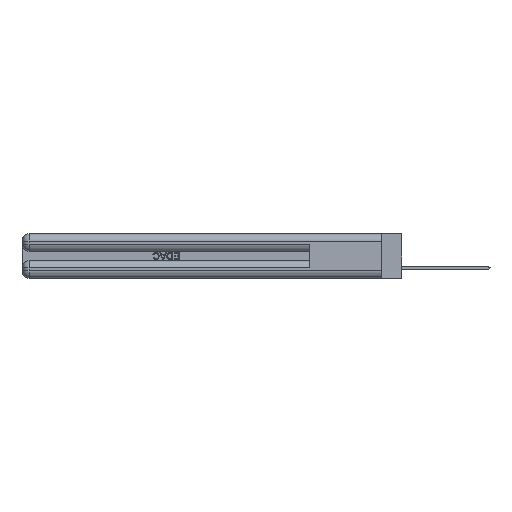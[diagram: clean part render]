
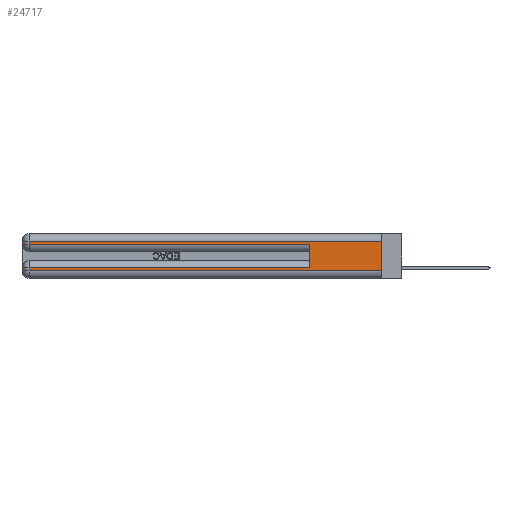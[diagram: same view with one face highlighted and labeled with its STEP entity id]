
A CAD part, left-side view. The second image highlights one B-rep face of the part: STEP entity #24717.
In plain terms, the highlighted planar face has unit normal (-1, 0, 0).
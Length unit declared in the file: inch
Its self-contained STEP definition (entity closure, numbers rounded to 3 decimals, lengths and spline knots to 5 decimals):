
#1017 = EDGE_CURVE ( 'NONE', #30338, #10760, #43060, .T. ) ;
#1776 = CARTESIAN_POINT ( 'NONE',  ( 0., 0., 0.31 ) ) ;
#2384 = CARTESIAN_POINT ( 'NONE',  ( 0., 0.6, 0.085 ) ) ;
#2623 = PLANE ( 'NONE',  #31251 ) ;
#4353 = VERTEX_POINT ( 'NONE', #27204 ) ;
#7682 = VECTOR ( 'NONE', #43996, 39.37008 ) ;
#8694 = VECTOR ( 'NONE', #31365, 39.37008 ) ;
#8896 = EDGE_LOOP ( 'NONE', ( #10251, #34363, #15253, #35273, #28475, #35552, #41959, #15795 ) ) ;
#10251 = ORIENTED_EDGE ( 'NONE', *, *, #39786, .F. ) ;
#10760 = VERTEX_POINT ( 'NONE', #42130 ) ;
#11633 = VERTEX_POINT ( 'NONE', #11650 ) ;
#11650 = CARTESIAN_POINT ( 'NONE',  ( 0., 0., 0.31 ) ) ;
#13659 = DIRECTION ( 'NONE',  ( 0., 0., -1. ) ) ;
#13691 = CARTESIAN_POINT ( 'NONE',  ( 0., 0., 0.085 ) ) ;
#13802 = VECTOR ( 'NONE', #17091, 39.37008 ) ;
#14340 = CARTESIAN_POINT ( 'NONE',  ( 0., 0., 0.06 ) ) ;
#14368 = CARTESIAN_POINT ( 'NONE',  ( 0., 0.6, 0.145 ) ) ;
#15253 = ORIENTED_EDGE ( 'NONE', *, *, #37008, .T. ) ;
#15402 = VECTOR ( 'NONE', #17909, 39.37008 ) ;
#15795 = ORIENTED_EDGE ( 'NONE', *, *, #37630, .T. ) ;
#16189 = LINE ( 'NONE', #1776, #31571 ) ;
#16237 = FACE_OUTER_BOUND ( 'NONE', #8896, .T. ) ;
#16579 = VECTOR ( 'NONE', #17939, 39.37008 ) ;
#16727 = CARTESIAN_POINT ( 'NONE',  ( 0., 0., 0.37 ) ) ;
#17091 = DIRECTION ( 'NONE',  ( 0., 1., 0. ) ) ;
#17909 = DIRECTION ( 'NONE',  ( 0., -1., 0. ) ) ;
#17939 = DIRECTION ( 'NONE',  ( 0., 0., 1. ) ) ;
#18750 = CARTESIAN_POINT ( 'NONE',  ( 0., 2.94, 0.37 ) ) ;
#20159 = VECTOR ( 'NONE', #25986, 39.37008 ) ;
#20836 = LINE ( 'NONE', #38506, #8694 ) ;
#21003 = EDGE_CURVE ( 'NONE', #36018, #32308, #36309, .T. ) ;
#21335 = CARTESIAN_POINT ( 'NONE',  ( 0., 2.94, 0.085 ) ) ;
#22274 = DIRECTION ( 'NONE',  ( 0., 0., -1. ) ) ;
#22298 = CARTESIAN_POINT ( 'NONE',  ( 0., 0., 0.285 ) ) ;
#22446 = CARTESIAN_POINT ( 'NONE',  ( 0., 2.94, 0.285 ) ) ;
#24717 = ADVANCED_FACE ( 'NONE', ( #16237 ), #2623, .F. ) ;
#24850 = VECTOR ( 'NONE', #22274, 39.37008 ) ;
#25943 = VERTEX_POINT ( 'NONE', #22446 ) ;
#25986 = DIRECTION ( 'NONE',  ( 0., 0., -1. ) ) ;
#27204 = CARTESIAN_POINT ( 'NONE',  ( 0., 2.94, 0.31 ) ) ;
#27719 = VERTEX_POINT ( 'NONE', #33353 ) ;
#27754 = EDGE_CURVE ( 'NONE', #25943, #32308, #35657, .T. ) ;
#28475 = ORIENTED_EDGE ( 'NONE', *, *, #21003, .F. ) ;
#28573 = CARTESIAN_POINT ( 'NONE',  ( 0., 2.94, 0.37 ) ) ;
#30338 = VERTEX_POINT ( 'NONE', #21335 ) ;
#31251 = AXIS2_PLACEMENT_3D ( 'NONE', #16727, #44143, #13659 ) ;
#31365 = DIRECTION ( 'NONE',  ( 0., 0., -1. ) ) ;
#31571 = VECTOR ( 'NONE', #36596, 39.37008 ) ;
#31593 = EDGE_CURVE ( 'NONE', #36018, #30338, #39519, .T. ) ;
#32308 = VERTEX_POINT ( 'NONE', #41978 ) ;
#33353 = CARTESIAN_POINT ( 'NONE',  ( 0., 0., 0.06 ) ) ;
#34186 = LINE ( 'NONE', #18750, #24850 ) ;
#34363 = ORIENTED_EDGE ( 'NONE', *, *, #43766, .T. ) ;
#35273 = ORIENTED_EDGE ( 'NONE', *, *, #27754, .T. ) ;
#35552 = ORIENTED_EDGE ( 'NONE', *, *, #31593, .T. ) ;
#35657 = LINE ( 'NONE', #22298, #7682 ) ;
#36018 = VERTEX_POINT ( 'NONE', #2384 ) ;
#36309 = LINE ( 'NONE', #14368, #16579 ) ;
#36596 = DIRECTION ( 'NONE',  ( 0., 1., 0. ) ) ;
#37008 = EDGE_CURVE ( 'NONE', #4353, #25943, #34186, .T. ) ;
#37630 = EDGE_CURVE ( 'NONE', #10760, #27719, #37937, .T. ) ;
#37937 = LINE ( 'NONE', #14340, #15402 ) ;
#38506 = CARTESIAN_POINT ( 'NONE',  ( 0., 0., 0.37 ) ) ;
#39519 = LINE ( 'NONE', #13691, #13802 ) ;
#39786 = EDGE_CURVE ( 'NONE', #11633, #27719, #20836, .T. ) ;
#41959 = ORIENTED_EDGE ( 'NONE', *, *, #1017, .T. ) ;
#41978 = CARTESIAN_POINT ( 'NONE',  ( 0., 0.6, 0.285 ) ) ;
#42130 = CARTESIAN_POINT ( 'NONE',  ( 0., 2.94, 0.06 ) ) ;
#43060 = LINE ( 'NONE', #28573, #20159 ) ;
#43766 = EDGE_CURVE ( 'NONE', #11633, #4353, #16189, .T. ) ;
#43996 = DIRECTION ( 'NONE',  ( 0., -1., 0. ) ) ;
#44143 = DIRECTION ( 'NONE',  ( 1., 0., 0. ) ) ;
